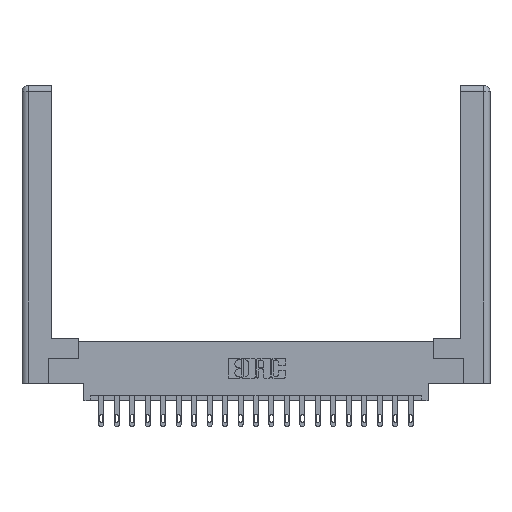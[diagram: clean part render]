
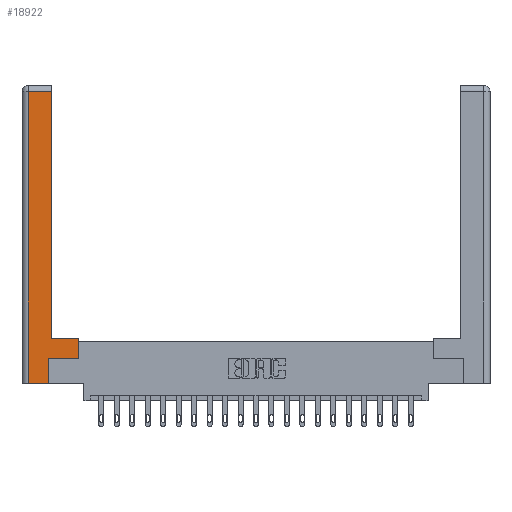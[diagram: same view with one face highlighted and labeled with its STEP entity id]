
A CAD part, top view. The second image highlights one B-rep face of the part: STEP entity #18922.
In plain terms, the highlighted planar face has unit normal (0, 0, 1).
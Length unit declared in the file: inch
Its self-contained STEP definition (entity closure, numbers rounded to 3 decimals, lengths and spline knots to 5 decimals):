
#258 = ORIENTED_EDGE ( 'NONE', *, *, #2704, .T. ) ;
#1376 = VECTOR ( 'NONE', #11586, 39.37008 ) ;
#1728 = VECTOR ( 'NONE', #12987, 39.37008 ) ;
#2641 = ORIENTED_EDGE ( 'NONE', *, *, #19667, .T. ) ;
#2704 = EDGE_CURVE ( 'NONE', #6426, #9334, #5608, .T. ) ;
#2764 = CARTESIAN_POINT ( 'NONE',  ( 0.265, 0.245, 0. ) ) ;
#2919 = AXIS2_PLACEMENT_3D ( 'NONE', #14891, #13499, #13436 ) ;
#3459 = PLANE ( 'NONE',  #2919 ) ;
#3515 = DIRECTION ( 'NONE',  ( -1., 0., 0. ) ) ;
#3918 = VERTEX_POINT ( 'NONE', #11086 ) ;
#4094 = VECTOR ( 'NONE', #12815, 39.37008 ) ;
#4804 = CARTESIAN_POINT ( 'NONE',  ( 0.295, 3., 0. ) ) ;
#4879 = VECTOR ( 'NONE', #20754, 39.37008 ) ;
#5142 = CARTESIAN_POINT ( 'NONE',  ( 0.565, 0.245, 0. ) ) ;
#5181 = CARTESIAN_POINT ( 'NONE',  ( 0.295, 0.45, 0. ) ) ;
#5608 = LINE ( 'NONE', #18826, #18724 ) ;
#5674 = LINE ( 'NONE', #7568, #4094 ) ;
#6426 = VERTEX_POINT ( 'NONE', #10474 ) ;
#6837 = CARTESIAN_POINT ( 'NONE',  ( 0.565, 0.45, 0. ) ) ;
#6952 = DIRECTION ( 'NONE',  ( 0., -1., 0. ) ) ;
#7014 = DIRECTION ( 'NONE',  ( 0., 1., 0. ) ) ;
#7089 = ORIENTED_EDGE ( 'NONE', *, *, #20470, .T. ) ;
#7568 = CARTESIAN_POINT ( 'NONE',  ( 0.565, 0.45, 0. ) ) ;
#8180 = CARTESIAN_POINT ( 'NONE',  ( 0.265, 0., 0. ) ) ;
#8657 = CARTESIAN_POINT ( 'NONE',  ( 0.295, 0.45, 0. ) ) ;
#8865 = ORIENTED_EDGE ( 'NONE', *, *, #11472, .T. ) ;
#8896 = FACE_OUTER_BOUND ( 'NONE', #11728, .T. ) ;
#8969 = ORIENTED_EDGE ( 'NONE', *, *, #9465, .T. ) ;
#9011 = LINE ( 'NONE', #4804, #1376 ) ;
#9334 = VERTEX_POINT ( 'NONE', #21606 ) ;
#9344 = VECTOR ( 'NONE', #7014, 39.37008 ) ;
#9465 = EDGE_CURVE ( 'NONE', #13011, #15039, #10147, .T. ) ;
#9709 = ORIENTED_EDGE ( 'NONE', *, *, #20204, .T. ) ;
#9841 = EDGE_CURVE ( 'NONE', #9334, #3918, #19838, .T. ) ;
#10038 = EDGE_CURVE ( 'NONE', #15151, #20467, #19283, .T. ) ;
#10147 = LINE ( 'NONE', #8657, #13311 ) ;
#10474 = CARTESIAN_POINT ( 'NONE',  ( 0.0615, 2.94, 0. ) ) ;
#10612 = CARTESIAN_POINT ( 'NONE',  ( 0.0615, 2.94, 0. ) ) ;
#11086 = CARTESIAN_POINT ( 'NONE',  ( 0.265, 0., 0. ) ) ;
#11472 = EDGE_CURVE ( 'NONE', #15039, #16797, #9011, .T. ) ;
#11586 = DIRECTION ( 'NONE',  ( 0., 1., 0. ) ) ;
#11728 = EDGE_LOOP ( 'NONE', ( #8865, #7089, #258, #13818, #2641, #15909, #9709, #8969 ) ) ;
#12815 = DIRECTION ( 'NONE',  ( 0., 1., 0. ) ) ;
#12987 = DIRECTION ( 'NONE',  ( 1., 0., 0. ) ) ;
#13011 = VERTEX_POINT ( 'NONE', #6837 ) ;
#13311 = VECTOR ( 'NONE', #3515, 39.37008 ) ;
#13436 = DIRECTION ( 'NONE',  ( -1., 0., 0. ) ) ;
#13499 = DIRECTION ( 'NONE',  ( 0., 0., -1. ) ) ;
#13818 = ORIENTED_EDGE ( 'NONE', *, *, #9841, .T. ) ;
#14340 = CARTESIAN_POINT ( 'NONE',  ( 0.565, 0.245, 0. ) ) ;
#14891 = CARTESIAN_POINT ( 'NONE',  ( 0., 0., 0. ) ) ;
#15039 = VERTEX_POINT ( 'NONE', #5181 ) ;
#15119 = LINE ( 'NONE', #10612, #20869 ) ;
#15151 = VERTEX_POINT ( 'NONE', #2764 ) ;
#15756 = DIRECTION ( 'NONE',  ( -1., 0., 0. ) ) ;
#15909 = ORIENTED_EDGE ( 'NONE', *, *, #10038, .T. ) ;
#16797 = VERTEX_POINT ( 'NONE', #19043 ) ;
#16984 = LINE ( 'NONE', #18812, #9344 ) ;
#18724 = VECTOR ( 'NONE', #6952, 39.37008 ) ;
#18812 = CARTESIAN_POINT ( 'NONE',  ( 0.265, 0.245, 0. ) ) ;
#18826 = CARTESIAN_POINT ( 'NONE',  ( 0.0615, 0., 0. ) ) ;
#18922 = ADVANCED_FACE ( 'NONE', ( #8896 ), #3459, .F. ) ;
#19043 = CARTESIAN_POINT ( 'NONE',  ( 0.295, 2.94, 0. ) ) ;
#19283 = LINE ( 'NONE', #14340, #4879 ) ;
#19667 = EDGE_CURVE ( 'NONE', #3918, #15151, #16984, .T. ) ;
#19838 = LINE ( 'NONE', #8180, #1728 ) ;
#20204 = EDGE_CURVE ( 'NONE', #20467, #13011, #5674, .T. ) ;
#20467 = VERTEX_POINT ( 'NONE', #5142 ) ;
#20470 = EDGE_CURVE ( 'NONE', #16797, #6426, #15119, .T. ) ;
#20754 = DIRECTION ( 'NONE',  ( 1., 0., 0. ) ) ;
#20869 = VECTOR ( 'NONE', #15756, 39.37008 ) ;
#21606 = CARTESIAN_POINT ( 'NONE',  ( 0.0615, 0., 0. ) ) ;
